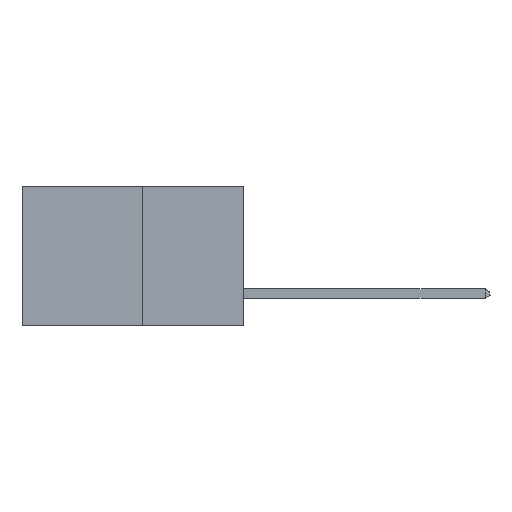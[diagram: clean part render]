
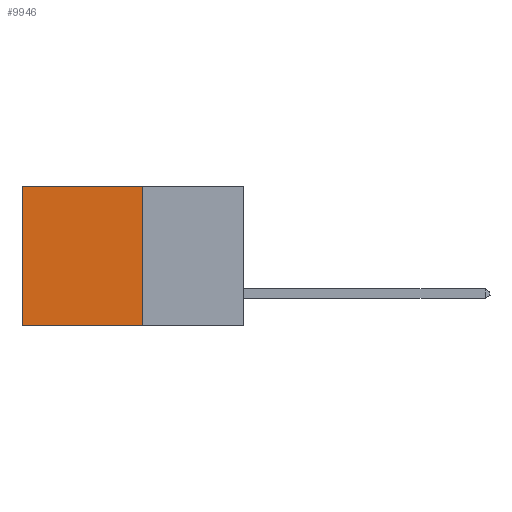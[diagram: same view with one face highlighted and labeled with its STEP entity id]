
A CAD part, left-side view. The second image highlights one B-rep face of the part: STEP entity #9946.
In plain terms, the highlighted planar face has unit normal (-1, 0, 0).
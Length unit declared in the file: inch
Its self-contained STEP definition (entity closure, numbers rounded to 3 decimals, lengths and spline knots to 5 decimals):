
#36 = DIRECTION ( 'NONE',  ( 0., 1., 0. ) ) ;
#160 = CARTESIAN_POINT ( 'NONE',  ( 0.277, 0.27, 0. ) ) ;
#358 = VERTEX_POINT ( 'NONE', #4354 ) ;
#892 = LINE ( 'NONE', #15529, #23174 ) ;
#1946 = DIRECTION ( 'NONE',  ( 0., 0., -1. ) ) ;
#3535 = VERTEX_POINT ( 'NONE', #15021 ) ;
#4354 = CARTESIAN_POINT ( 'NONE',  ( 0.277, 0.59, 0. ) ) ;
#4618 = DIRECTION ( 'NONE',  ( 0., 0., -1. ) ) ;
#4643 = EDGE_CURVE ( 'NONE', #21019, #358, #19492, .T. ) ;
#6987 = DIRECTION ( 'NONE',  ( 1., 0., 0. ) ) ;
#8495 = CARTESIAN_POINT ( 'NONE',  ( 0.277, 0.27, -0.37 ) ) ;
#9085 = VERTEX_POINT ( 'NONE', #26031 ) ;
#9776 = EDGE_LOOP ( 'NONE', ( #22389, #10128, #24328, #12628 ) ) ;
#9946 = ADVANCED_FACE ( 'NONE', ( #20926 ), #26463, .F. ) ;
#10128 = ORIENTED_EDGE ( 'NONE', *, *, #12291, .F. ) ;
#12291 = EDGE_CURVE ( 'NONE', #9085, #3535, #20121, .T. ) ;
#12628 = ORIENTED_EDGE ( 'NONE', *, *, #4643, .T. ) ;
#12817 = CARTESIAN_POINT ( 'NONE',  ( 0.277, 0.27, -0.37 ) ) ;
#13667 = VECTOR ( 'NONE', #36, 39.37008 ) ;
#15021 = CARTESIAN_POINT ( 'NONE',  ( 0.277, 0.59, -0.37 ) ) ;
#15065 = VECTOR ( 'NONE', #1946, 39.37008 ) ;
#15529 = CARTESIAN_POINT ( 'NONE',  ( 0.277, 0.59, -0.37 ) ) ;
#16751 = EDGE_CURVE ( 'NONE', #21019, #9085, #25236, .T. ) ;
#19492 = LINE ( 'NONE', #160, #13667 ) ;
#20099 = CARTESIAN_POINT ( 'NONE',  ( 0.277, 0.27, -0.37 ) ) ;
#20121 = LINE ( 'NONE', #8495, #25815 ) ;
#20926 = FACE_OUTER_BOUND ( 'NONE', #9776, .T. ) ;
#21019 = VERTEX_POINT ( 'NONE', #23574 ) ;
#22289 = DIRECTION ( 'NONE',  ( 0., 0., -1. ) ) ;
#22389 = ORIENTED_EDGE ( 'NONE', *, *, #24787, .T. ) ;
#23174 = VECTOR ( 'NONE', #4618, 39.37008 ) ;
#23574 = CARTESIAN_POINT ( 'NONE',  ( 0.277, 0.27, 0. ) ) ;
#23690 = DIRECTION ( 'NONE',  ( 0., 1., 0. ) ) ;
#24328 = ORIENTED_EDGE ( 'NONE', *, *, #16751, .F. ) ;
#24787 = EDGE_CURVE ( 'NONE', #358, #3535, #892, .T. ) ;
#25236 = LINE ( 'NONE', #12817, #15065 ) ;
#25815 = VECTOR ( 'NONE', #23690, 39.37008 ) ;
#26031 = CARTESIAN_POINT ( 'NONE',  ( 0.277, 0.27, -0.37 ) ) ;
#26463 = PLANE ( 'NONE',  #27815 ) ;
#27815 = AXIS2_PLACEMENT_3D ( 'NONE', #20099, #6987, #22289 ) ;
